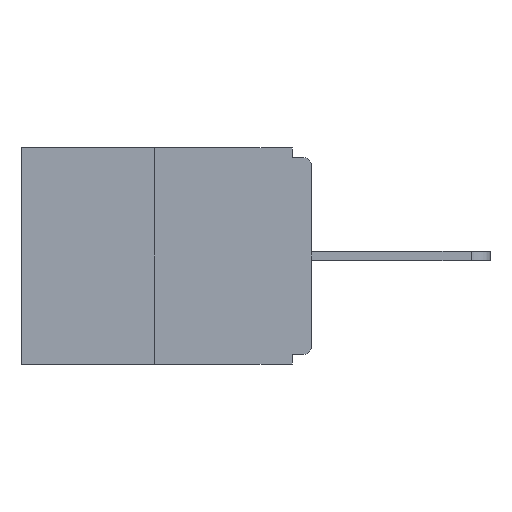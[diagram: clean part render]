
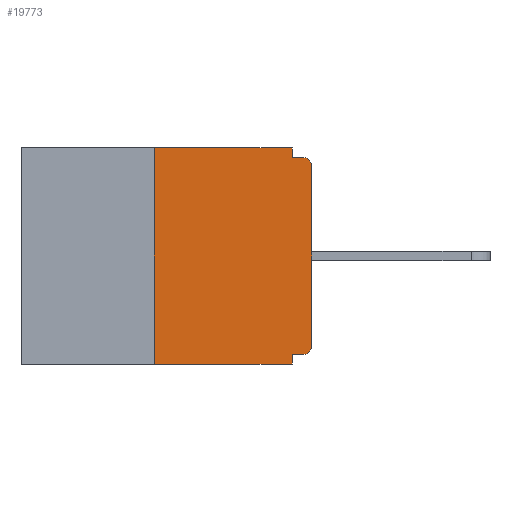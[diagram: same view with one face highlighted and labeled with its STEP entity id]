
A CAD part, left-side view. The second image highlights one B-rep face of the part: STEP entity #19773.
In plain terms, the highlighted planar face has unit normal (-1, 0, 0).
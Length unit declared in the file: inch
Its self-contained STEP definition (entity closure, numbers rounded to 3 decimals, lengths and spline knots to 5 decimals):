
#581 = PLANE ( 'NONE',  #5795 ) ;
#754 = CARTESIAN_POINT ( 'NONE',  ( 0., 0., -0.313 ) ) ;
#788 = CARTESIAN_POINT ( 'NONE',  ( 0., 0.015, -0.313 ) ) ;
#1065 = DIRECTION ( 'NONE',  ( 0., 0., -1. ) ) ;
#1082 = DIRECTION ( 'NONE',  ( -1., 0., 0. ) ) ;
#1299 = AXIS2_PLACEMENT_3D ( 'NONE', #788, #1082, #1065 ) ;
#1695 = ORIENTED_EDGE ( 'NONE', *, *, #6270, .F. ) ;
#2013 = CARTESIAN_POINT ( 'NONE',  ( 0., 0.031, -0.328 ) ) ;
#2293 = ORIENTED_EDGE ( 'NONE', *, *, #18273, .T. ) ;
#2397 = VERTEX_POINT ( 'NONE', #754 ) ;
#3322 = CARTESIAN_POINT ( 'NONE',  ( 0., 0.031, 0. ) ) ;
#3501 = EDGE_CURVE ( 'NONE', #18431, #2397, #13062, .T. ) ;
#3973 = CARTESIAN_POINT ( 'NONE',  ( 0., 0.46, 0. ) ) ;
#4210 = CARTESIAN_POINT ( 'NONE',  ( 0., 0.031, -0.343 ) ) ;
#4293 = CARTESIAN_POINT ( 'NONE',  ( 0., 0.031, -0.015 ) ) ;
#4483 = LINE ( 'NONE', #4210, #8304 ) ;
#4611 = VECTOR ( 'NONE', #11242, 39.37008 ) ;
#4621 = CARTESIAN_POINT ( 'NONE',  ( 0., 0.25, 0. ) ) ;
#4847 = CARTESIAN_POINT ( 'NONE',  ( 0., 0.015, -0.03 ) ) ;
#5356 = LINE ( 'NONE', #14690, #9150 ) ;
#5642 = DIRECTION ( 'NONE',  ( 0., 0., -1. ) ) ;
#5656 = LINE ( 'NONE', #17272, #4611 ) ;
#5795 = AXIS2_PLACEMENT_3D ( 'NONE', #3973, #15055, #5642 ) ;
#6270 = EDGE_CURVE ( 'NONE', #11299, #19553, #15443, .T. ) ;
#6437 = CARTESIAN_POINT ( 'NONE',  ( 0., 0., -0.015 ) ) ;
#6444 = EDGE_LOOP ( 'NONE', ( #1695, #12787, #19204, #12119, #18529, #13310, #12140, #2293, #12383, #18339 ) ) ;
#6505 = DIRECTION ( 'NONE',  ( 0., -1., 0. ) ) ;
#6507 = DIRECTION ( 'NONE',  ( 0., 0., -1. ) ) ;
#6580 = CARTESIAN_POINT ( 'NONE',  ( 0., 0.031, 0. ) ) ;
#6883 = VECTOR ( 'NONE', #17912, 39.37008 ) ;
#6990 = EDGE_CURVE ( 'NONE', #9194, #11299, #15177, .T. ) ;
#7178 = CARTESIAN_POINT ( 'NONE',  ( 0., 0.25, 0. ) ) ;
#7536 = DIRECTION ( 'NONE',  ( 0., 0., -1. ) ) ;
#8304 = VECTOR ( 'NONE', #7536, 39.37008 ) ;
#8516 = DIRECTION ( 'NONE',  ( 0., 1., 0. ) ) ;
#8536 = CARTESIAN_POINT ( 'NONE',  ( 0., 0.015, -0.328 ) ) ;
#9150 = VECTOR ( 'NONE', #8516, 39.37008 ) ;
#9194 = VERTEX_POINT ( 'NONE', #12718 ) ;
#9650 = FACE_OUTER_BOUND ( 'NONE', #6444, .T. ) ;
#9713 = EDGE_CURVE ( 'NONE', #19303, #16150, #18628, .T. ) ;
#9773 = DIRECTION ( 'NONE',  ( 0., 0., -1. ) ) ;
#11242 = DIRECTION ( 'NONE',  ( 0., 0., 1. ) ) ;
#11291 = VECTOR ( 'NONE', #16323, 39.37008 ) ;
#11299 = VERTEX_POINT ( 'NONE', #4621 ) ;
#11341 = VECTOR ( 'NONE', #15545, 39.37008 ) ;
#11919 = EDGE_CURVE ( 'NONE', #2397, #15147, #5656, .T. ) ;
#12119 = ORIENTED_EDGE ( 'NONE', *, *, #12903, .F. ) ;
#12140 = ORIENTED_EDGE ( 'NONE', *, *, #11919, .T. ) ;
#12383 = ORIENTED_EDGE ( 'NONE', *, *, #9713, .F. ) ;
#12426 = AXIS2_PLACEMENT_3D ( 'NONE', #4847, #15841, #6507 ) ;
#12718 = CARTESIAN_POINT ( 'NONE',  ( 0., 0.25, -0.343 ) ) ;
#12787 = ORIENTED_EDGE ( 'NONE', *, *, #6990, .F. ) ;
#12903 = EDGE_CURVE ( 'NONE', #13443, #16707, #4483, .T. ) ;
#13062 = CIRCLE ( 'NONE', #1299, 0.015 ) ;
#13310 = ORIENTED_EDGE ( 'NONE', *, *, #3501, .T. ) ;
#13443 = VERTEX_POINT ( 'NONE', #2013 ) ;
#14522 = VECTOR ( 'NONE', #9773, 39.37008 ) ;
#14690 = CARTESIAN_POINT ( 'NONE',  ( 0., 0., -0.328 ) ) ;
#14723 = CARTESIAN_POINT ( 'NONE',  ( 0., 0., -0.03 ) ) ;
#14808 = CARTESIAN_POINT ( 'NONE',  ( 0., 0.015, -0.015 ) ) ;
#14812 = CARTESIAN_POINT ( 'NONE',  ( 0., 0.46, -0.343 ) ) ;
#15055 = DIRECTION ( 'NONE',  ( 1., 0., 0. ) ) ;
#15147 = VERTEX_POINT ( 'NONE', #14723 ) ;
#15177 = LINE ( 'NONE', #7178, #6883 ) ;
#15393 = LINE ( 'NONE', #14812, #11291 ) ;
#15443 = LINE ( 'NONE', #20347, #11341 ) ;
#15545 = DIRECTION ( 'NONE',  ( 0., -1., 0. ) ) ;
#15841 = DIRECTION ( 'NONE',  ( -1., 0., 0. ) ) ;
#16150 = VERTEX_POINT ( 'NONE', #14808 ) ;
#16323 = DIRECTION ( 'NONE',  ( 0., -1., 0. ) ) ;
#16707 = VERTEX_POINT ( 'NONE', #19400 ) ;
#17272 = CARTESIAN_POINT ( 'NONE',  ( 0., 0., 0. ) ) ;
#17883 = EDGE_CURVE ( 'NONE', #9194, #16707, #15393, .T. ) ;
#17912 = DIRECTION ( 'NONE',  ( 0., 0., 1. ) ) ;
#18166 = VECTOR ( 'NONE', #6505, 39.37008 ) ;
#18273 = EDGE_CURVE ( 'NONE', #15147, #16150, #19986, .T. ) ;
#18339 = ORIENTED_EDGE ( 'NONE', *, *, #19535, .F. ) ;
#18431 = VERTEX_POINT ( 'NONE', #8536 ) ;
#18529 = ORIENTED_EDGE ( 'NONE', *, *, #20214, .F. ) ;
#18535 = LINE ( 'NONE', #6580, #14522 ) ;
#18628 = LINE ( 'NONE', #6437, #18166 ) ;
#19204 = ORIENTED_EDGE ( 'NONE', *, *, #17883, .T. ) ;
#19303 = VERTEX_POINT ( 'NONE', #4293 ) ;
#19400 = CARTESIAN_POINT ( 'NONE',  ( 0., 0.031, -0.343 ) ) ;
#19535 = EDGE_CURVE ( 'NONE', #19553, #19303, #18535, .T. ) ;
#19553 = VERTEX_POINT ( 'NONE', #3322 ) ;
#19773 = ADVANCED_FACE ( 'NONE', ( #9650 ), #581, .F. ) ;
#19986 = CIRCLE ( 'NONE', #12426, 0.015 ) ;
#20214 = EDGE_CURVE ( 'NONE', #18431, #13443, #5356, .T. ) ;
#20347 = CARTESIAN_POINT ( 'NONE',  ( 0., 0.46, 0. ) ) ;
